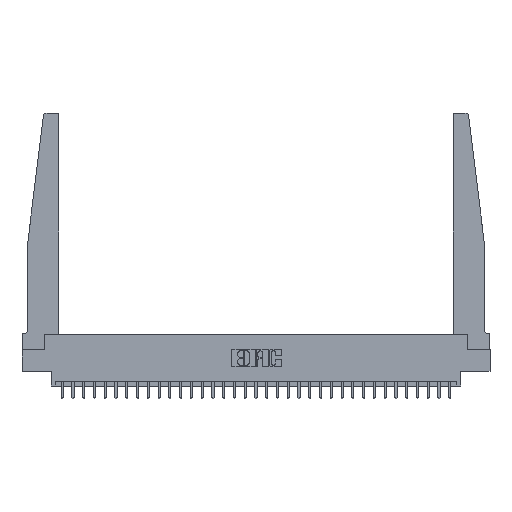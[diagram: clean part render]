
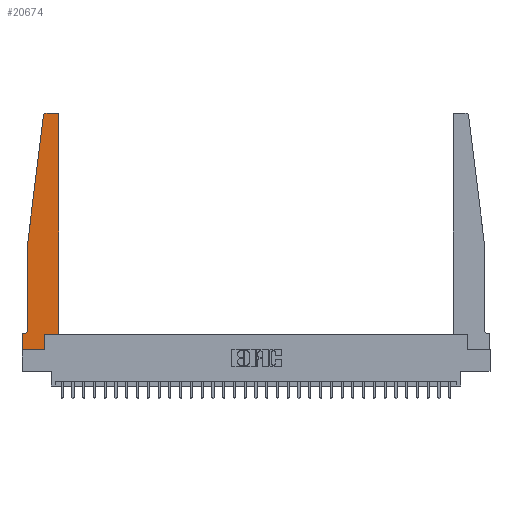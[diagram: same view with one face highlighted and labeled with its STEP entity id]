
A CAD part, top view. The second image highlights one B-rep face of the part: STEP entity #20674.
In plain terms, the highlighted planar face has unit normal (0, 0, 1).
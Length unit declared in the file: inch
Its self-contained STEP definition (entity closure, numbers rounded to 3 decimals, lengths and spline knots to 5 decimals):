
#95 = VERTEX_POINT ( 'NONE', #872 ) ;
#872 = CARTESIAN_POINT ( 'NONE',  ( 0.2605, 0.18, 0.37 ) ) ;
#1191 = VECTOR ( 'NONE', #13068, 39.37008 ) ;
#1303 = ORIENTED_EDGE ( 'NONE', *, *, #28444, .T. ) ;
#1306 = EDGE_CURVE ( 'NONE', #29187, #7118, #22261, .T. ) ;
#2171 = CARTESIAN_POINT ( 'NONE',  ( 0.425, 2.72, 0.37 ) ) ;
#2603 = VERTEX_POINT ( 'NONE', #22382 ) ;
#2898 = CARTESIAN_POINT ( 'NONE',  ( 0.27653, 2.75, 0.37 ) ) ;
#2905 = CARTESIAN_POINT ( 'NONE',  ( 0.065, 1.25, 0.37 ) ) ;
#3164 = DIRECTION ( 'NONE',  ( 0., 1., 0. ) ) ;
#3366 = DIRECTION ( 'NONE',  ( 0., -1., 0. ) ) ;
#3673 = CARTESIAN_POINT ( 'NONE',  ( 0., 0., 0.37 ) ) ;
#3802 = CARTESIAN_POINT ( 'NONE',  ( 0.065, 1.25, 0.37 ) ) ;
#4063 = EDGE_CURVE ( 'NONE', #8948, #16486, #18444, .T. ) ;
#4729 = CARTESIAN_POINT ( 'NONE',  ( 0.395, 2.75, 0.37 ) ) ;
#5383 = VECTOR ( 'NONE', #3366, 39.37008 ) ;
#5393 = VECTOR ( 'NONE', #26225, 39.37008 ) ;
#5535 = VECTOR ( 'NONE', #6003, 39.37008 ) ;
#5768 = PLANE ( 'NONE',  #8904 ) ;
#5968 = LINE ( 'NONE', #3673, #1191 ) ;
#5995 = EDGE_CURVE ( 'NONE', #12740, #13948, #23410, .T. ) ;
#6003 = DIRECTION ( 'NONE',  ( 1., 0., 0. ) ) ;
#6079 = CARTESIAN_POINT ( 'NONE',  ( 0.25, 2.75, 0.37 ) ) ;
#6956 = LINE ( 'NONE', #19119, #5393 ) ;
#7118 = VERTEX_POINT ( 'NONE', #13145 ) ;
#7614 = EDGE_CURVE ( 'NONE', #7118, #8948, #26331, .T. ) ;
#7622 = ORIENTED_EDGE ( 'NONE', *, *, #7614, .T. ) ;
#7771 = ORIENTED_EDGE ( 'NONE', *, *, #21765, .T. ) ;
#7915 = FACE_OUTER_BOUND ( 'NONE', #23250, .T. ) ;
#8020 = VERTEX_POINT ( 'NONE', #16683 ) ;
#8569 = DIRECTION ( 'NONE',  ( -0.122, -0.992, 0. ) ) ;
#8774 = VECTOR ( 'NONE', #16164, 39.37008 ) ;
#8904 = AXIS2_PLACEMENT_3D ( 'NONE', #12696, #26289, #15152 ) ;
#8948 = VERTEX_POINT ( 'NONE', #10401 ) ;
#9231 = ORIENTED_EDGE ( 'NONE', *, *, #21657, .T. ) ;
#9879 = VECTOR ( 'NONE', #20564, 39.37008 ) ;
#10275 = VERTEX_POINT ( 'NONE', #2898 ) ;
#10401 = CARTESIAN_POINT ( 'NONE',  ( 0.065, 0.2375, 0.37 ) ) ;
#10839 = EDGE_CURVE ( 'NONE', #13948, #95, #21636, .T. ) ;
#11585 = CARTESIAN_POINT ( 'NONE',  ( 0.065, 0.1875, 0.37 ) ) ;
#12077 = CARTESIAN_POINT ( 'NONE',  ( 0., 0., 0.37 ) ) ;
#12188 = ORIENTED_EDGE ( 'NONE', *, *, #5995, .T. ) ;
#12696 = CARTESIAN_POINT ( 'NONE',  ( 0., 0.1875, 0.37 ) ) ;
#12740 = VERTEX_POINT ( 'NONE', #27889 ) ;
#13068 = DIRECTION ( 'NONE',  ( 0., -1., 0. ) ) ;
#13091 = VECTOR ( 'NONE', #16219, 39.37008 ) ;
#13145 = CARTESIAN_POINT ( 'NONE',  ( 0.065, 1.25, 0.37 ) ) ;
#13701 = DIRECTION ( 'NONE',  ( 1., 0., 0. ) ) ;
#13948 = VERTEX_POINT ( 'NONE', #17817 ) ;
#15063 = EDGE_CURVE ( 'NONE', #10275, #29187, #20703, .T. ) ;
#15152 = DIRECTION ( 'NONE',  ( 1., 0., 0. ) ) ;
#15566 = ORIENTED_EDGE ( 'NONE', *, *, #20760, .T. ) ;
#16138 = CARTESIAN_POINT ( 'NONE',  ( 0.27653, 2.72, 0.37 ) ) ;
#16164 = DIRECTION ( 'NONE',  ( -1., 0., 0. ) ) ;
#16193 = CARTESIAN_POINT ( 'NONE',  ( 0.395, 2.72, 0.37 ) ) ;
#16219 = DIRECTION ( 'NONE',  ( 1., 0., 0. ) ) ;
#16486 = VERTEX_POINT ( 'NONE', #20667 ) ;
#16683 = CARTESIAN_POINT ( 'NONE',  ( 0., 0.1875, 0.37 ) ) ;
#17185 = CARTESIAN_POINT ( 'NONE',  ( 0.24675, 2.72367, 0.37 ) ) ;
#17433 = CARTESIAN_POINT ( 'NONE',  ( 0.015, 0.2375, 0.37 ) ) ;
#17591 = DIRECTION ( 'NONE',  ( -1., 0., 0. ) ) ;
#17817 = CARTESIAN_POINT ( 'NONE',  ( 0.2605, 0., 0.37 ) ) ;
#17856 = ORIENTED_EDGE ( 'NONE', *, *, #1306, .T. ) ;
#18196 = EDGE_CURVE ( 'NONE', #16486, #8020, #27882, .T. ) ;
#18444 = CIRCLE ( 'NONE', #23309, 0.05 ) ;
#18834 = DIRECTION ( 'NONE',  ( 0., 0., 1. ) ) ;
#19080 = VERTEX_POINT ( 'NONE', #4729 ) ;
#19119 = CARTESIAN_POINT ( 'NONE',  ( 0.425, 0.18, 0.37 ) ) ;
#19436 = ORIENTED_EDGE ( 'NONE', *, *, #15063, .T. ) ;
#19824 = VERTEX_POINT ( 'NONE', #2171 ) ;
#20564 = DIRECTION ( 'NONE',  ( -1., 0., 0. ) ) ;
#20667 = CARTESIAN_POINT ( 'NONE',  ( 0.015, 0.1875, 0.37 ) ) ;
#20674 = ADVANCED_FACE ( 'NONE', ( #7915 ), #5768, .T. ) ;
#20703 = CIRCLE ( 'NONE', #26957, 0.03 ) ;
#20760 = EDGE_CURVE ( 'NONE', #19080, #10275, #27190, .T. ) ;
#21636 = LINE ( 'NONE', #24165, #22146 ) ;
#21657 = EDGE_CURVE ( 'NONE', #19824, #19080, #25662, .T. ) ;
#21675 = VECTOR ( 'NONE', #8569, 39.37008 ) ;
#21765 = EDGE_CURVE ( 'NONE', #2603, #19824, #6956, .T. ) ;
#22146 = VECTOR ( 'NONE', #3164, 39.37008 ) ;
#22261 = LINE ( 'NONE', #3802, #21675 ) ;
#22382 = CARTESIAN_POINT ( 'NONE',  ( 0.425, 0.18, 0.37 ) ) ;
#23250 = EDGE_LOOP ( 'NONE', ( #15566, #19436, #17856, #7622, #24443, #29421, #1303, #12188, #25132, #26147, #7771, #9231 ) ) ;
#23309 = AXIS2_PLACEMENT_3D ( 'NONE', #17433, #29137, #17591 ) ;
#23387 = DIRECTION ( 'NONE',  ( 1., 0., 0. ) ) ;
#23410 = LINE ( 'NONE', #12077, #13091 ) ;
#24165 = CARTESIAN_POINT ( 'NONE',  ( 0.2605, 0.18, 0.37 ) ) ;
#24443 = ORIENTED_EDGE ( 'NONE', *, *, #4063, .T. ) ;
#25132 = ORIENTED_EDGE ( 'NONE', *, *, #10839, .T. ) ;
#25662 = CIRCLE ( 'NONE', #26132, 0.03 ) ;
#26132 = AXIS2_PLACEMENT_3D ( 'NONE', #16193, #18834, #23387 ) ;
#26147 = ORIENTED_EDGE ( 'NONE', *, *, #26903, .T. ) ;
#26225 = DIRECTION ( 'NONE',  ( 0., 1., 0. ) ) ;
#26289 = DIRECTION ( 'NONE',  ( 0., 0., 1. ) ) ;
#26331 = LINE ( 'NONE', #2905, #5383 ) ;
#26903 = EDGE_CURVE ( 'NONE', #95, #2603, #28776, .T. ) ;
#26957 = AXIS2_PLACEMENT_3D ( 'NONE', #16138, #27559, #13701 ) ;
#26967 = CARTESIAN_POINT ( 'NONE',  ( 0.425, 0.18, 0.37 ) ) ;
#27190 = LINE ( 'NONE', #6079, #9879 ) ;
#27559 = DIRECTION ( 'NONE',  ( 0., 0., 1. ) ) ;
#27882 = LINE ( 'NONE', #11585, #8774 ) ;
#27889 = CARTESIAN_POINT ( 'NONE',  ( 0., 0., 0.37 ) ) ;
#28444 = EDGE_CURVE ( 'NONE', #8020, #12740, #5968, .T. ) ;
#28776 = LINE ( 'NONE', #26967, #5535 ) ;
#29137 = DIRECTION ( 'NONE',  ( 0., 0., -1. ) ) ;
#29187 = VERTEX_POINT ( 'NONE', #17185 ) ;
#29421 = ORIENTED_EDGE ( 'NONE', *, *, #18196, .T. ) ;
